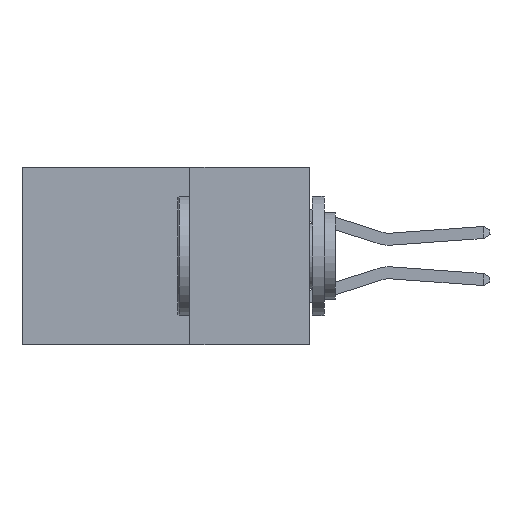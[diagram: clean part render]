
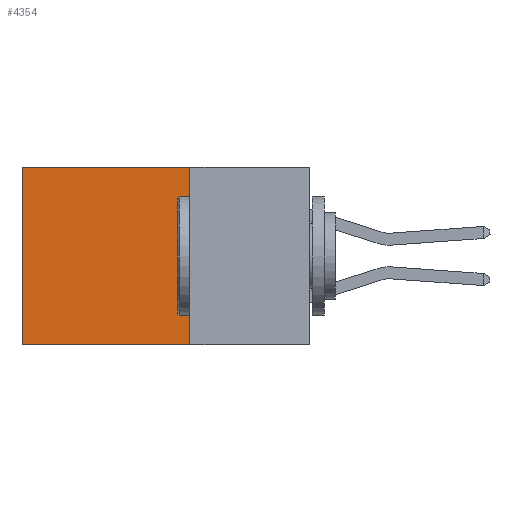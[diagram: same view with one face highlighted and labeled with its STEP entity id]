
A CAD part, left-side view. The second image highlights one B-rep face of the part: STEP entity #4354.
In plain terms, the highlighted planar face has unit normal (-1, 0, 0).
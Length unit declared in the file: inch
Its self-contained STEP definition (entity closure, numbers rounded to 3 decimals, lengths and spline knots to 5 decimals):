
#16 = LINE ( 'NONE', #2864, #3219 ) ;
#280 = ORIENTED_EDGE ( 'NONE', *, *, #8883, .T. ) ;
#350 = ORIENTED_EDGE ( 'NONE', *, *, #9575, .F. ) ;
#393 = ORIENTED_EDGE ( 'NONE', *, *, #8190, .F. ) ;
#407 = ORIENTED_EDGE ( 'NONE', *, *, #12406, .T. ) ;
#655 = DIRECTION ( 'NONE',  ( 0., 1., 0. ) ) ;
#770 = CARTESIAN_POINT ( 'NONE',  ( 0.2615, 0.25, -0.37 ) ) ;
#1219 = AXIS2_PLACEMENT_3D ( 'NONE', #5900, #5853, #5839 ) ;
#1619 = LINE ( 'NONE', #11563, #10567 ) ;
#2864 = CARTESIAN_POINT ( 'NONE',  ( 0.2615, 0.25, -0.37 ) ) ;
#3167 = LINE ( 'NONE', #770, #14646 ) ;
#3219 = VECTOR ( 'NONE', #4960, 39.37008 ) ;
#3507 = DIRECTION ( 'NONE',  ( 0., 0., -1. ) ) ;
#3566 = CARTESIAN_POINT ( 'NONE',  ( 0.2615, 0.6, -0.37 ) ) ;
#4354 = ADVANCED_FACE ( 'NONE', ( #13684 ), #6007, .F. ) ;
#4960 = DIRECTION ( 'NONE',  ( 0., 0., -1. ) ) ;
#5838 = VECTOR ( 'NONE', #3507, 39.37008 ) ;
#5839 = DIRECTION ( 'NONE',  ( 0., 0., -1. ) ) ;
#5853 = DIRECTION ( 'NONE',  ( 1., 0., 0. ) ) ;
#5895 = VERTEX_POINT ( 'NONE', #9970 ) ;
#5900 = CARTESIAN_POINT ( 'NONE',  ( 0.2615, 0.25, -0.37 ) ) ;
#6007 = PLANE ( 'NONE',  #1219 ) ;
#7799 = EDGE_LOOP ( 'NONE', ( #280, #350, #393, #407 ) ) ;
#8159 = CARTESIAN_POINT ( 'NONE',  ( 0.2615, 0.25, 0. ) ) ;
#8190 = EDGE_CURVE ( 'NONE', #11711, #5895, #16, .T. ) ;
#8764 = VERTEX_POINT ( 'NONE', #10641 ) ;
#8883 = EDGE_CURVE ( 'NONE', #9091, #8764, #9560, .T. ) ;
#9091 = VERTEX_POINT ( 'NONE', #10531 ) ;
#9560 = LINE ( 'NONE', #3566, #5838 ) ;
#9575 = EDGE_CURVE ( 'NONE', #5895, #8764, #3167, .T. ) ;
#9970 = CARTESIAN_POINT ( 'NONE',  ( 0.2615, 0.25, -0.37 ) ) ;
#10531 = CARTESIAN_POINT ( 'NONE',  ( 0.2615, 0.6, 0. ) ) ;
#10567 = VECTOR ( 'NONE', #11640, 39.37008 ) ;
#10641 = CARTESIAN_POINT ( 'NONE',  ( 0.2615, 0.6, -0.37 ) ) ;
#11563 = CARTESIAN_POINT ( 'NONE',  ( 0.2615, 0.25, 0. ) ) ;
#11640 = DIRECTION ( 'NONE',  ( 0., 1., 0. ) ) ;
#11711 = VERTEX_POINT ( 'NONE', #8159 ) ;
#12406 = EDGE_CURVE ( 'NONE', #11711, #9091, #1619, .T. ) ;
#13684 = FACE_OUTER_BOUND ( 'NONE', #7799, .T. ) ;
#14646 = VECTOR ( 'NONE', #655, 39.37008 ) ;
